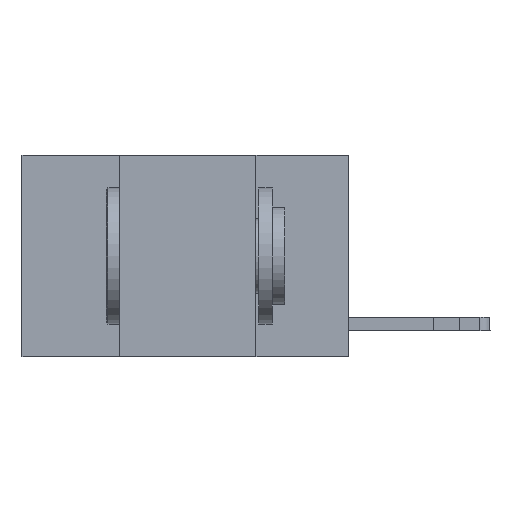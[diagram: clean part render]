
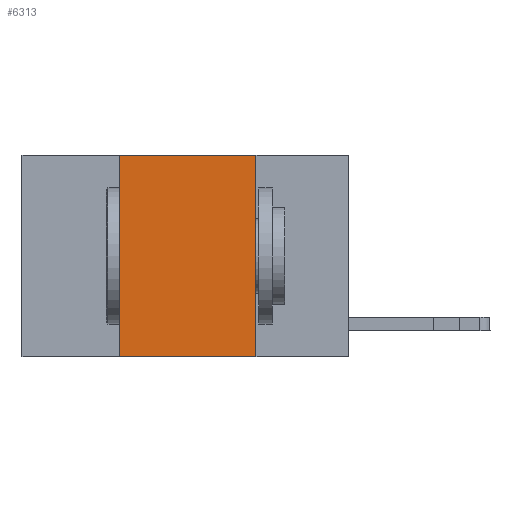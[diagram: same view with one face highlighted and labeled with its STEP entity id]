
A CAD part, left-side view. The second image highlights one B-rep face of the part: STEP entity #6313.
In plain terms, the highlighted planar face has unit normal (-1, 0, 0).
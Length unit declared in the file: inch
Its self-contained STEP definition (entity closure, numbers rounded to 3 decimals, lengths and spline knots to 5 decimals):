
#1165 = DIRECTION ( 'NONE',  ( 0., -1., 0. ) ) ;
#1977 = VERTEX_POINT ( 'NONE', #2011 ) ;
#2011 = CARTESIAN_POINT ( 'NONE',  ( 0., 0.42, -0.37 ) ) ;
#2468 = ORIENTED_EDGE ( 'NONE', *, *, #20840, .F. ) ;
#3401 = VECTOR ( 'NONE', #8942, 39.37008 ) ;
#3647 = FACE_OUTER_BOUND ( 'NONE', #18281, .T. ) ;
#5371 = PLANE ( 'NONE',  #9059 ) ;
#5696 = VERTEX_POINT ( 'NONE', #11158 ) ;
#5736 = CARTESIAN_POINT ( 'NONE',  ( 0., 0.17, -0.37 ) ) ;
#5802 = LINE ( 'NONE', #10980, #3401 ) ;
#6313 = ADVANCED_FACE ( 'NONE', ( #3647 ), #5371, .F. ) ;
#8180 = CARTESIAN_POINT ( 'NONE',  ( 0., 0.6, 0. ) ) ;
#8543 = LINE ( 'NONE', #19777, #20678 ) ;
#8624 = DIRECTION ( 'NONE',  ( 1., 0., 0. ) ) ;
#8752 = CARTESIAN_POINT ( 'NONE',  ( 0., 0.6, -0.37 ) ) ;
#8942 = DIRECTION ( 'NONE',  ( 0., 0., 1. ) ) ;
#8976 = LINE ( 'NONE', #8752, #15793 ) ;
#9059 = AXIS2_PLACEMENT_3D ( 'NONE', #17163, #8624, #11966 ) ;
#9887 = VECTOR ( 'NONE', #18442, 39.37008 ) ;
#9927 = DIRECTION ( 'NONE',  ( 0., 0., -1. ) ) ;
#10980 = CARTESIAN_POINT ( 'NONE',  ( 0., 0.42, 0. ) ) ;
#11158 = CARTESIAN_POINT ( 'NONE',  ( 0., 0.42, 0. ) ) ;
#11245 = ORIENTED_EDGE ( 'NONE', *, *, #20538, .T. ) ;
#11966 = DIRECTION ( 'NONE',  ( 0., 0., -1. ) ) ;
#14010 = EDGE_CURVE ( 'NONE', #5696, #19871, #14654, .T. ) ;
#14654 = LINE ( 'NONE', #8180, #9887 ) ;
#15106 = ORIENTED_EDGE ( 'NONE', *, *, #19757, .F. ) ;
#15578 = VERTEX_POINT ( 'NONE', #5736 ) ;
#15793 = VECTOR ( 'NONE', #1165, 39.37008 ) ;
#16042 = CARTESIAN_POINT ( 'NONE',  ( 0., 0.17, 0. ) ) ;
#17163 = CARTESIAN_POINT ( 'NONE',  ( 0., 0.6, 0. ) ) ;
#18281 = EDGE_LOOP ( 'NONE', ( #2468, #20706, #15106, #11245 ) ) ;
#18442 = DIRECTION ( 'NONE',  ( 0., -1., 0. ) ) ;
#19757 = EDGE_CURVE ( 'NONE', #1977, #5696, #5802, .T. ) ;
#19777 = CARTESIAN_POINT ( 'NONE',  ( 0., 0.17, 0. ) ) ;
#19871 = VERTEX_POINT ( 'NONE', #16042 ) ;
#20538 = EDGE_CURVE ( 'NONE', #1977, #15578, #8976, .T. ) ;
#20678 = VECTOR ( 'NONE', #9927, 39.37008 ) ;
#20706 = ORIENTED_EDGE ( 'NONE', *, *, #14010, .F. ) ;
#20840 = EDGE_CURVE ( 'NONE', #19871, #15578, #8543, .T. ) ;
